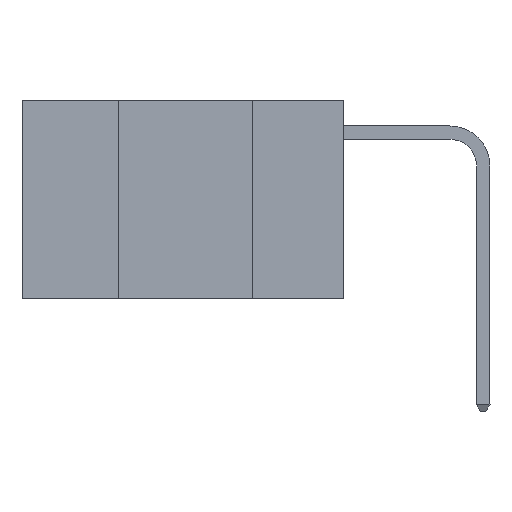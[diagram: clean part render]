
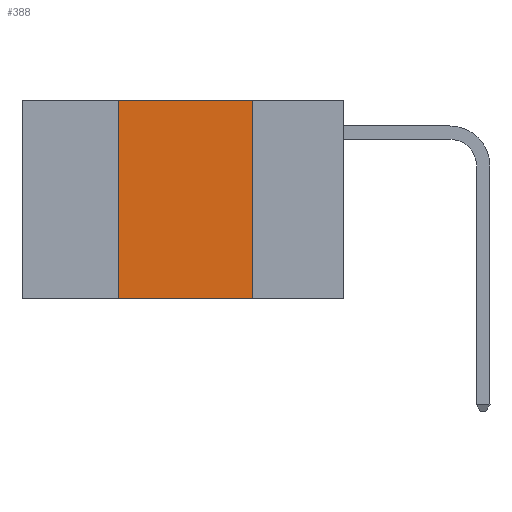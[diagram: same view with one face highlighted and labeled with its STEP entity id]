
A CAD part, left-side view. The second image highlights one B-rep face of the part: STEP entity #388.
In plain terms, the highlighted planar face has unit normal (-1, 0, 0).
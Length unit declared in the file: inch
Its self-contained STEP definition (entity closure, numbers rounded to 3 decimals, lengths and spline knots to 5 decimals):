
#159 = PLANE ( 'NONE',  #2944 ) ;
#388 = ADVANCED_FACE ( 'NONE', ( #10947 ), #159, .F. ) ;
#462 = EDGE_CURVE ( 'NONE', #7561, #8014, #12032, .T. ) ;
#606 = CARTESIAN_POINT ( 'NONE',  ( 0., 0.6, -0.37 ) ) ;
#660 = VECTOR ( 'NONE', #10615, 39.37008 ) ;
#830 = ORIENTED_EDGE ( 'NONE', *, *, #462, .F. ) ;
#1191 = ORIENTED_EDGE ( 'NONE', *, *, #10698, .F. ) ;
#2061 = VECTOR ( 'NONE', #2595, 39.37008 ) ;
#2349 = VECTOR ( 'NONE', #3716, 39.37008 ) ;
#2495 = CARTESIAN_POINT ( 'NONE',  ( 0., 0.17, -0.37 ) ) ;
#2595 = DIRECTION ( 'NONE',  ( 0., -1., 0. ) ) ;
#2944 = AXIS2_PLACEMENT_3D ( 'NONE', #9928, #4079, #6995 ) ;
#3309 = CARTESIAN_POINT ( 'NONE',  ( 0., 0.42, 0. ) ) ;
#3716 = DIRECTION ( 'NONE',  ( 0., -1., 0. ) ) ;
#3942 = ORIENTED_EDGE ( 'NONE', *, *, #8574, .F. ) ;
#4079 = DIRECTION ( 'NONE',  ( 1., 0., 0. ) ) ;
#4590 = VECTOR ( 'NONE', #7178, 39.37008 ) ;
#4890 = CARTESIAN_POINT ( 'NONE',  ( 0., 0.6, 0. ) ) ;
#6076 = VERTEX_POINT ( 'NONE', #2495 ) ;
#6247 = CARTESIAN_POINT ( 'NONE',  ( 0., 0.42, -0.37 ) ) ;
#6715 = CARTESIAN_POINT ( 'NONE',  ( 0., 0.17, 0. ) ) ;
#6995 = DIRECTION ( 'NONE',  ( 0., 0., -1. ) ) ;
#7099 = EDGE_CURVE ( 'NONE', #7561, #6076, #11328, .T. ) ;
#7178 = DIRECTION ( 'NONE',  ( 0., 0., 1. ) ) ;
#7561 = VERTEX_POINT ( 'NONE', #6247 ) ;
#8014 = VERTEX_POINT ( 'NONE', #8932 ) ;
#8241 = ORIENTED_EDGE ( 'NONE', *, *, #7099, .T. ) ;
#8574 = EDGE_CURVE ( 'NONE', #11042, #6076, #11576, .T. ) ;
#8687 = LINE ( 'NONE', #4890, #2349 ) ;
#8932 = CARTESIAN_POINT ( 'NONE',  ( 0., 0.42, 0. ) ) ;
#9928 = CARTESIAN_POINT ( 'NONE',  ( 0., 0.6, 0. ) ) ;
#10615 = DIRECTION ( 'NONE',  ( 0., 0., -1. ) ) ;
#10698 = EDGE_CURVE ( 'NONE', #8014, #11042, #8687, .T. ) ;
#10859 = EDGE_LOOP ( 'NONE', ( #3942, #1191, #830, #8241 ) ) ;
#10947 = FACE_OUTER_BOUND ( 'NONE', #10859, .T. ) ;
#11042 = VERTEX_POINT ( 'NONE', #11200 ) ;
#11200 = CARTESIAN_POINT ( 'NONE',  ( 0., 0.17, 0. ) ) ;
#11328 = LINE ( 'NONE', #606, #2061 ) ;
#11576 = LINE ( 'NONE', #6715, #660 ) ;
#12032 = LINE ( 'NONE', #3309, #4590 ) ;
